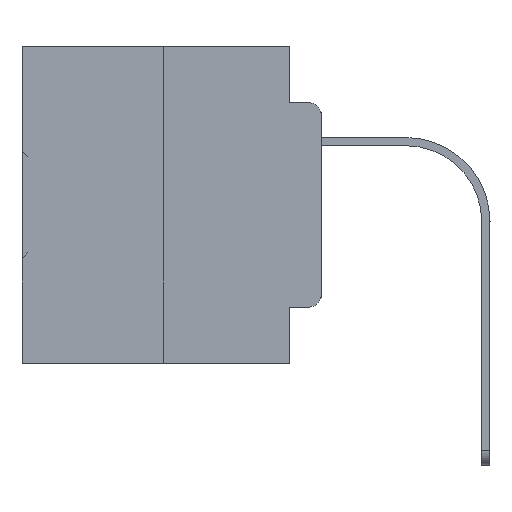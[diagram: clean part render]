
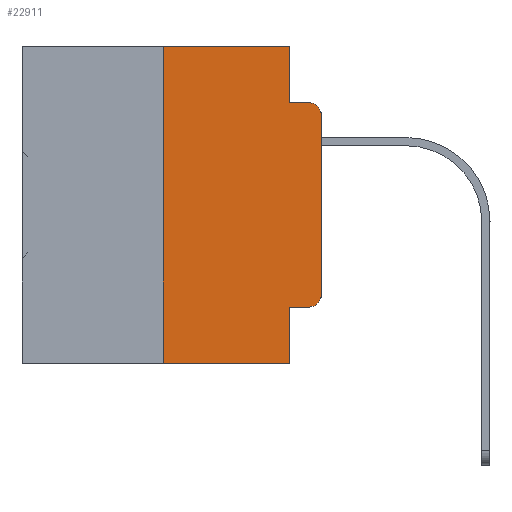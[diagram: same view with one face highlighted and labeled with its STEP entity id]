
A CAD part, left-side view. The second image highlights one B-rep face of the part: STEP entity #22911.
In plain terms, the highlighted planar face has unit normal (-1, 0, 0).
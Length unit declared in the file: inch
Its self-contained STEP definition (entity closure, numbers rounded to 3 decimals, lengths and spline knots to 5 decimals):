
#44 = ORIENTED_EDGE ( 'NONE', *, *, #18192, .T. ) ;
#430 = CARTESIAN_POINT ( 'NONE',  ( 0., 0.473, 0. ) ) ;
#1569 = CARTESIAN_POINT ( 'NONE',  ( 0., 0.051, -0.4115 ) ) ;
#2588 = VECTOR ( 'NONE', #25220, 39.37008 ) ;
#2739 = CARTESIAN_POINT ( 'NONE',  ( 0., 0.051, 0. ) ) ;
#3124 = EDGE_CURVE ( 'NONE', #25087, #13377, #34172, .T. ) ;
#3279 = DIRECTION ( 'NONE',  ( 0., 0., -1. ) ) ;
#4316 = CARTESIAN_POINT ( 'NONE',  ( 0., 0.473, -0.5 ) ) ;
#4584 = LINE ( 'NONE', #14125, #29416 ) ;
#5009 = EDGE_CURVE ( 'NONE', #10990, #30925, #17360, .T. ) ;
#5320 = CARTESIAN_POINT ( 'NONE',  ( 0., 0.051, 0. ) ) ;
#6432 = VERTEX_POINT ( 'NONE', #10812 ) ;
#6603 = EDGE_CURVE ( 'NONE', #6432, #20484, #12557, .T. ) ;
#6790 = VECTOR ( 'NONE', #12377, 39.37008 ) ;
#7212 = LINE ( 'NONE', #12831, #23196 ) ;
#7270 = EDGE_CURVE ( 'NONE', #31716, #10990, #32438, .T. ) ;
#7517 = DIRECTION ( 'NONE',  ( 0., 0., -1. ) ) ;
#8691 = VECTOR ( 'NONE', #11110, 39.37008 ) ;
#9672 = DIRECTION ( 'NONE',  ( 0., 0., 1. ) ) ;
#10024 = DIRECTION ( 'NONE',  ( 0., -1., 0. ) ) ;
#10812 = CARTESIAN_POINT ( 'NONE',  ( 0., 0.25, -0.5 ) ) ;
#10990 = VERTEX_POINT ( 'NONE', #24598 ) ;
#11110 = DIRECTION ( 'NONE',  ( 0., -1., 0. ) ) ;
#11185 = AXIS2_PLACEMENT_3D ( 'NONE', #11686, #32905, #3279 ) ;
#11686 = CARTESIAN_POINT ( 'NONE',  ( 0., 0.02, -0.3915 ) ) ;
#12377 = DIRECTION ( 'NONE',  ( 0., -1., 0. ) ) ;
#12557 = LINE ( 'NONE', #4316, #6790 ) ;
#12831 = CARTESIAN_POINT ( 'NONE',  ( 0., 0.051, -0.0885 ) ) ;
#12918 = CARTESIAN_POINT ( 'NONE',  ( 0., 0.051, -0.0885 ) ) ;
#13078 = DIRECTION ( 'NONE',  ( 0., 0., -1. ) ) ;
#13377 = VERTEX_POINT ( 'NONE', #12918 ) ;
#13579 = ORIENTED_EDGE ( 'NONE', *, *, #5009, .T. ) ;
#13859 = CARTESIAN_POINT ( 'NONE',  ( 0., 0.02, -0.0885 ) ) ;
#14125 = CARTESIAN_POINT ( 'NONE',  ( 0., 0.25, 0. ) ) ;
#14600 = FACE_OUTER_BOUND ( 'NONE', #19335, .T. ) ;
#15169 = CARTESIAN_POINT ( 'NONE',  ( 0., 0., 0. ) ) ;
#15801 = VERTEX_POINT ( 'NONE', #13859 ) ;
#16579 = VECTOR ( 'NONE', #13078, 39.37008 ) ;
#17216 = ORIENTED_EDGE ( 'NONE', *, *, #23484, .F. ) ;
#17360 = CIRCLE ( 'NONE', #11185, 0.02 ) ;
#17504 = ORIENTED_EDGE ( 'NONE', *, *, #21587, .F. ) ;
#17576 = PLANE ( 'NONE',  #24919 ) ;
#17878 = CARTESIAN_POINT ( 'NONE',  ( 0., 0.051, -0.4115 ) ) ;
#18192 = EDGE_CURVE ( 'NONE', #30925, #27579, #28487, .T. ) ;
#19335 = EDGE_LOOP ( 'NONE', ( #44, #30342, #34622, #33676, #28755, #17504, #32115, #17216, #26277, #13579 ) ) ;
#20484 = VERTEX_POINT ( 'NONE', #34046 ) ;
#20495 = EDGE_CURVE ( 'NONE', #13377, #15801, #7212, .T. ) ;
#21416 = VECTOR ( 'NONE', #7517, 39.37008 ) ;
#21587 = EDGE_CURVE ( 'NONE', #6432, #22073, #4584, .T. ) ;
#22073 = VERTEX_POINT ( 'NONE', #28049 ) ;
#22911 = ADVANCED_FACE ( 'NONE', ( #14600 ), #17576, .F. ) ;
#23196 = VECTOR ( 'NONE', #10024, 39.37008 ) ;
#23251 = CARTESIAN_POINT ( 'NONE',  ( 0., 0., -0.3915 ) ) ;
#23396 = CARTESIAN_POINT ( 'NONE',  ( 0., 0.02, -0.1085 ) ) ;
#23484 = EDGE_CURVE ( 'NONE', #31716, #20484, #24102, .T. ) ;
#23767 = EDGE_CURVE ( 'NONE', #27579, #15801, #26627, .T. ) ;
#23847 = AXIS2_PLACEMENT_3D ( 'NONE', #23396, #25499, #25319 ) ;
#24102 = LINE ( 'NONE', #2739, #16579 ) ;
#24423 = LINE ( 'NONE', #430, #8691 ) ;
#24598 = CARTESIAN_POINT ( 'NONE',  ( 0., 0.02, -0.4115 ) ) ;
#24919 = AXIS2_PLACEMENT_3D ( 'NONE', #30727, #31243, #27923 ) ;
#25087 = VERTEX_POINT ( 'NONE', #5320 ) ;
#25220 = DIRECTION ( 'NONE',  ( 0., -1., 0. ) ) ;
#25319 = DIRECTION ( 'NONE',  ( 0., 0., -1. ) ) ;
#25349 = EDGE_CURVE ( 'NONE', #22073, #25087, #24423, .T. ) ;
#25499 = DIRECTION ( 'NONE',  ( -1., 0., 0. ) ) ;
#25844 = DIRECTION ( 'NONE',  ( 0., 0., 1. ) ) ;
#25935 = CARTESIAN_POINT ( 'NONE',  ( 0., 0.051, 0. ) ) ;
#26277 = ORIENTED_EDGE ( 'NONE', *, *, #7270, .T. ) ;
#26627 = CIRCLE ( 'NONE', #23847, 0.02 ) ;
#27579 = VERTEX_POINT ( 'NONE', #31070 ) ;
#27923 = DIRECTION ( 'NONE',  ( 0., 0., -1. ) ) ;
#28049 = CARTESIAN_POINT ( 'NONE',  ( 0., 0.25, 0. ) ) ;
#28487 = LINE ( 'NONE', #15169, #33018 ) ;
#28755 = ORIENTED_EDGE ( 'NONE', *, *, #25349, .F. ) ;
#29416 = VECTOR ( 'NONE', #9672, 39.37008 ) ;
#30342 = ORIENTED_EDGE ( 'NONE', *, *, #23767, .T. ) ;
#30727 = CARTESIAN_POINT ( 'NONE',  ( 0., 0.473, 0. ) ) ;
#30925 = VERTEX_POINT ( 'NONE', #23251 ) ;
#31070 = CARTESIAN_POINT ( 'NONE',  ( 0., 0., -0.1085 ) ) ;
#31243 = DIRECTION ( 'NONE',  ( 1., 0., 0. ) ) ;
#31716 = VERTEX_POINT ( 'NONE', #17878 ) ;
#32115 = ORIENTED_EDGE ( 'NONE', *, *, #6603, .T. ) ;
#32438 = LINE ( 'NONE', #1569, #2588 ) ;
#32905 = DIRECTION ( 'NONE',  ( -1., 0., 0. ) ) ;
#33018 = VECTOR ( 'NONE', #25844, 39.37008 ) ;
#33676 = ORIENTED_EDGE ( 'NONE', *, *, #3124, .F. ) ;
#34046 = CARTESIAN_POINT ( 'NONE',  ( 0., 0.051, -0.5 ) ) ;
#34172 = LINE ( 'NONE', #25935, #21416 ) ;
#34622 = ORIENTED_EDGE ( 'NONE', *, *, #20495, .F. ) ;
